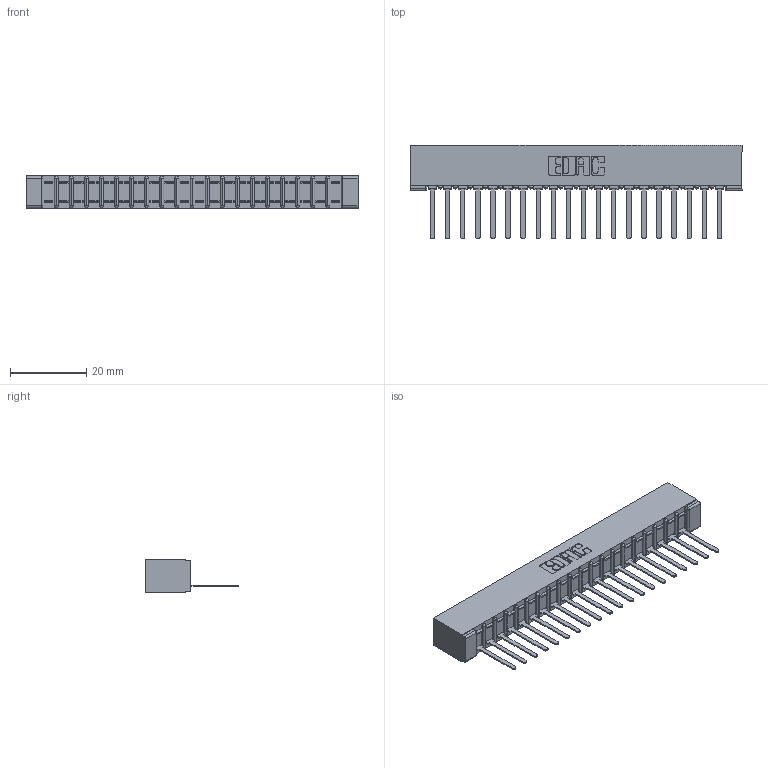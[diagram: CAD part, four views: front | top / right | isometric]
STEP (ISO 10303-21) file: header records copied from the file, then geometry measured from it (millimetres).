
FILE_DESCRIPTION (( 'STEP AP203' ), '1' );
FILE_NAME ('357-020-541-101.STEP', '2019-09-16T22:18:31', ( '' ), ( '' ), 'SwSTEP 2.0', 'SolidWorks 2016', '' );
FILE_SCHEMA (( 'CONFIG_CONTROL_DESIGN' ));
Length unit declared in the file: inch
Products named in the file (3): 307 Part_No Mounting Lugs; 357-020-541-101; 307-290-002_541
Assembly tree (21 placements, depth 2):
  357-020-541-101
    307 Part_No Mounting Lugs
    307-290-002_541  x20
Bounding box: 87.12 x 24.59 x 8.71 mm (x, y, z)
Volume: 6049.3 mm3; surface area: 11739.6 mm2
Topology: 21 solids, 21 shells, 1611 faces, 4939 edges, 3234 vertices
Faces by surface type: plane 966, cylinder 603, sphere 42
Entity records: 20298 total; most frequent: CARTESIAN_POINT 3420, ORIENTED_EDGE 3410, DIRECTION 3331, EDGE_CURVE 1705, VECTOR 1297, LINE 1297, VERTEX_POINT 1106, AXIS2_PLACEMENT_3D 1017
